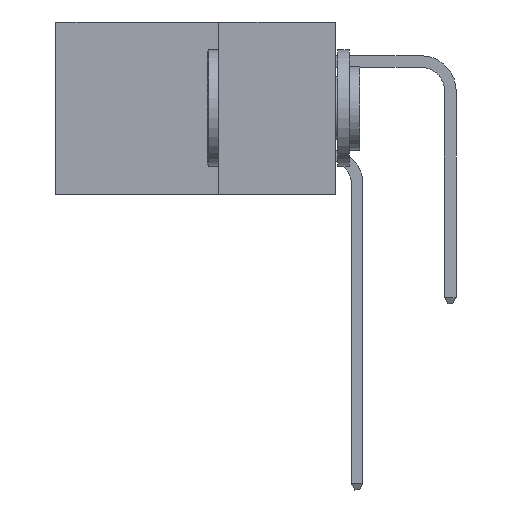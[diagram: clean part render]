
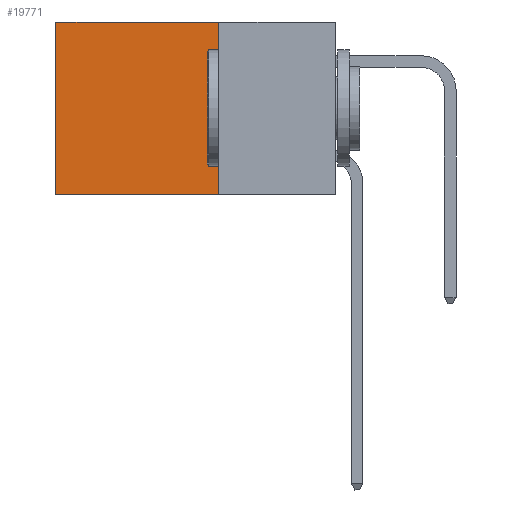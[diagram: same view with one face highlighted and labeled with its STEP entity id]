
A CAD part, left-side view. The second image highlights one B-rep face of the part: STEP entity #19771.
In plain terms, the highlighted planar face has unit normal (-1, 0, 0).
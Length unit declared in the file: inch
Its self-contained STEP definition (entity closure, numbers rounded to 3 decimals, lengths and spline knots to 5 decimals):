
#211 = CARTESIAN_POINT ( 'NONE',  ( 0.2875, 0.25, 0. ) ) ;
#618 = DIRECTION ( 'NONE',  ( 0., 1., 0. ) ) ;
#1119 = DIRECTION ( 'NONE',  ( 0., 0., -1. ) ) ;
#1463 = PLANE ( 'NONE',  #22784 ) ;
#2021 = VERTEX_POINT ( 'NONE', #13188 ) ;
#2287 = ORIENTED_EDGE ( 'NONE', *, *, #3360, .T. ) ;
#3234 = CARTESIAN_POINT ( 'NONE',  ( 0.2875, 0.25, 0. ) ) ;
#3271 = DIRECTION ( 'NONE',  ( 0., 1., 0. ) ) ;
#3360 = EDGE_CURVE ( 'NONE', #21560, #19343, #23395, .T. ) ;
#4650 = EDGE_CURVE ( 'NONE', #2021, #11713, #8237, .T. ) ;
#4734 = VECTOR ( 'NONE', #618, 39.37008 ) ;
#5332 = DIRECTION ( 'NONE',  ( 0., 0., -1. ) ) ;
#8237 = LINE ( 'NONE', #18102, #16897 ) ;
#10400 = LINE ( 'NONE', #16603, #15330 ) ;
#11713 = VERTEX_POINT ( 'NONE', #19819 ) ;
#12956 = DIRECTION ( 'NONE',  ( 0., 0., -1. ) ) ;
#13109 = CARTESIAN_POINT ( 'NONE',  ( 0.2875, 0.25, 0. ) ) ;
#13188 = CARTESIAN_POINT ( 'NONE',  ( 0.2875, 0.25, -0.37 ) ) ;
#13362 = ORIENTED_EDGE ( 'NONE', *, *, #24149, .T. ) ;
#14426 = VECTOR ( 'NONE', #1119, 39.37008 ) ;
#15330 = VECTOR ( 'NONE', #12956, 39.37008 ) ;
#16101 = EDGE_CURVE ( 'NONE', #21560, #2021, #10400, .T. ) ;
#16438 = DIRECTION ( 'NONE',  ( 1., 0., 0. ) ) ;
#16603 = CARTESIAN_POINT ( 'NONE',  ( 0.2875, 0.25, 0. ) ) ;
#16897 = VECTOR ( 'NONE', #3271, 39.37008 ) ;
#18102 = CARTESIAN_POINT ( 'NONE',  ( 0.2875, 0.25, -0.37 ) ) ;
#19340 = LINE ( 'NONE', #19728, #14426 ) ;
#19343 = VERTEX_POINT ( 'NONE', #24048 ) ;
#19728 = CARTESIAN_POINT ( 'NONE',  ( 0.2875, 0.6, 0. ) ) ;
#19771 = ADVANCED_FACE ( 'NONE', ( #21259 ), #1463, .F. ) ;
#19819 = CARTESIAN_POINT ( 'NONE',  ( 0.2875, 0.6, -0.37 ) ) ;
#19989 = ORIENTED_EDGE ( 'NONE', *, *, #4650, .F. ) ;
#21259 = FACE_OUTER_BOUND ( 'NONE', #23677, .T. ) ;
#21560 = VERTEX_POINT ( 'NONE', #13109 ) ;
#22784 = AXIS2_PLACEMENT_3D ( 'NONE', #3234, #16438, #5332 ) ;
#23395 = LINE ( 'NONE', #211, #4734 ) ;
#23677 = EDGE_LOOP ( 'NONE', ( #13362, #19989, #24134, #2287 ) ) ;
#24048 = CARTESIAN_POINT ( 'NONE',  ( 0.2875, 0.6, 0. ) ) ;
#24134 = ORIENTED_EDGE ( 'NONE', *, *, #16101, .F. ) ;
#24149 = EDGE_CURVE ( 'NONE', #19343, #11713, #19340, .T. ) ;
